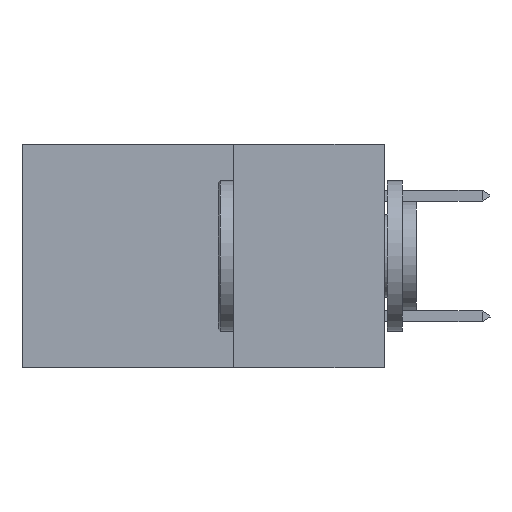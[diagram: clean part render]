
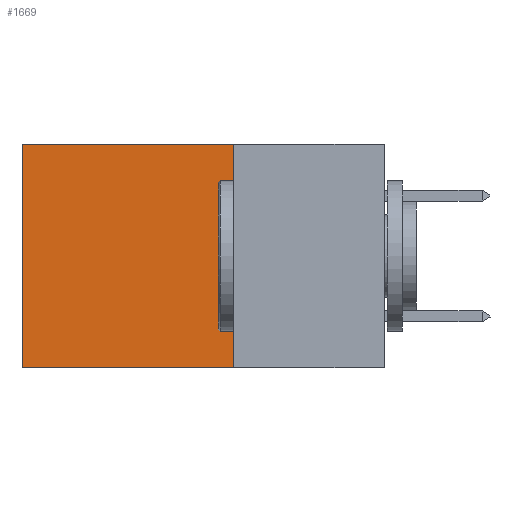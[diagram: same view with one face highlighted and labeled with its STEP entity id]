
A CAD part, left-side view. The second image highlights one B-rep face of the part: STEP entity #1669.
In plain terms, the highlighted planar face has unit normal (-1, 0, 0).
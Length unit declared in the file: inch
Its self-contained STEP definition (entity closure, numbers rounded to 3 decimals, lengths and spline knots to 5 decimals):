
#15 = EDGE_CURVE ( 'NONE', #4391, #12459, #7012, .T. ) ;
#616 = EDGE_CURVE ( 'NONE', #2362, #12459, #1357, .T. ) ;
#1037 = PLANE ( 'NONE',  #9339 ) ;
#1357 = LINE ( 'NONE', #10069, #2950 ) ;
#1669 = ADVANCED_FACE ( 'NONE', ( #7833 ), #1037, .F. ) ;
#2362 = VERTEX_POINT ( 'NONE', #8567 ) ;
#2459 = CARTESIAN_POINT ( 'NONE',  ( 0.2875, 0.25, -0.37 ) ) ;
#2467 = ORIENTED_EDGE ( 'NONE', *, *, #15, .F. ) ;
#2950 = VECTOR ( 'NONE', #8204, 39.37008 ) ;
#2972 = CARTESIAN_POINT ( 'NONE',  ( 0.2875, 0.25, -0.37 ) ) ;
#3088 = EDGE_CURVE ( 'NONE', #10045, #4391, #7010, .T. ) ;
#4046 = DIRECTION ( 'NONE',  ( 0., 1., 0. ) ) ;
#4391 = VERTEX_POINT ( 'NONE', #2459 ) ;
#5218 = VECTOR ( 'NONE', #4046, 39.37008 ) ;
#5463 = VECTOR ( 'NONE', #6072, 39.37008 ) ;
#5625 = ORIENTED_EDGE ( 'NONE', *, *, #3088, .F. ) ;
#6072 = DIRECTION ( 'NONE',  ( 0., 1., 0. ) ) ;
#6241 = CARTESIAN_POINT ( 'NONE',  ( 0.2875, 0.25, 0. ) ) ;
#7003 = EDGE_CURVE ( 'NONE', #10045, #2362, #12688, .T. ) ;
#7010 = LINE ( 'NONE', #7109, #9356 ) ;
#7012 = LINE ( 'NONE', #2972, #5463 ) ;
#7109 = CARTESIAN_POINT ( 'NONE',  ( 0.2875, 0.25, 0. ) ) ;
#7833 = FACE_OUTER_BOUND ( 'NONE', #10697, .T. ) ;
#7898 = CARTESIAN_POINT ( 'NONE',  ( 0.2875, 0.6, -0.37 ) ) ;
#8204 = DIRECTION ( 'NONE',  ( 0., 0., -1. ) ) ;
#8567 = CARTESIAN_POINT ( 'NONE',  ( 0.2875, 0.6, 0. ) ) ;
#9339 = AXIS2_PLACEMENT_3D ( 'NONE', #12097, #10036, #12920 ) ;
#9356 = VECTOR ( 'NONE', #9981, 39.37008 ) ;
#9981 = DIRECTION ( 'NONE',  ( 0., 0., -1. ) ) ;
#10000 = CARTESIAN_POINT ( 'NONE',  ( 0.2875, 0.25, 0. ) ) ;
#10036 = DIRECTION ( 'NONE',  ( 1., 0., 0. ) ) ;
#10045 = VERTEX_POINT ( 'NONE', #6241 ) ;
#10069 = CARTESIAN_POINT ( 'NONE',  ( 0.2875, 0.6, 0. ) ) ;
#10697 = EDGE_LOOP ( 'NONE', ( #12386, #2467, #5625, #12488 ) ) ;
#12097 = CARTESIAN_POINT ( 'NONE',  ( 0.2875, 0.25, 0. ) ) ;
#12386 = ORIENTED_EDGE ( 'NONE', *, *, #616, .T. ) ;
#12459 = VERTEX_POINT ( 'NONE', #7898 ) ;
#12488 = ORIENTED_EDGE ( 'NONE', *, *, #7003, .T. ) ;
#12688 = LINE ( 'NONE', #10000, #5218 ) ;
#12920 = DIRECTION ( 'NONE',  ( 0., 0., -1. ) ) ;
